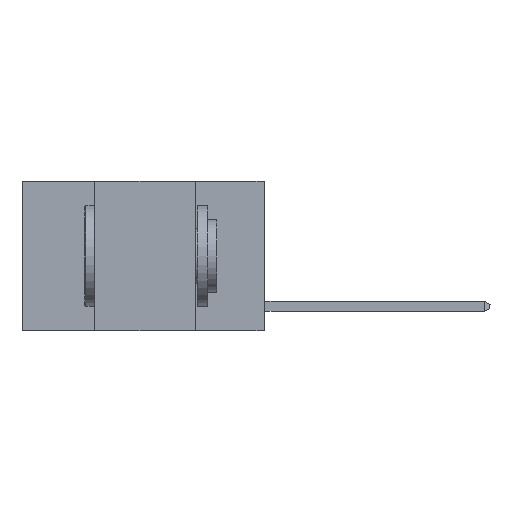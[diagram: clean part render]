
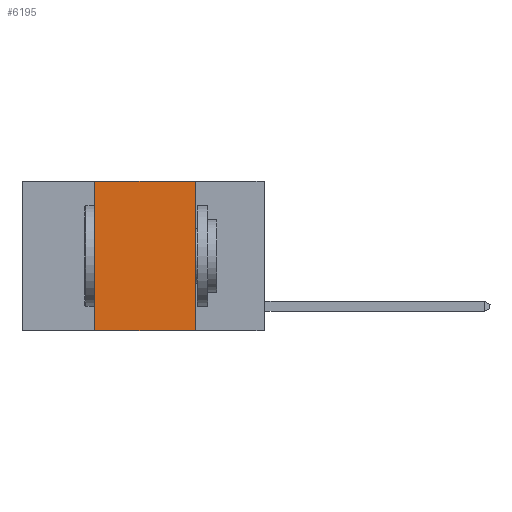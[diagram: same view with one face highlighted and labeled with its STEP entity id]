
A CAD part, left-side view. The second image highlights one B-rep face of the part: STEP entity #6195.
In plain terms, the highlighted planar face has unit normal (-1, 0, 0).
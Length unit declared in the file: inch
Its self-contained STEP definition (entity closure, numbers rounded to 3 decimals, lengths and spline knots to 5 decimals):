
#592 = CARTESIAN_POINT ( 'NONE',  ( 0., 0.17, 0. ) ) ;
#2072 = AXIS2_PLACEMENT_3D ( 'NONE', #7834, #9591, #21299 ) ;
#2615 = EDGE_CURVE ( 'NONE', #9611, #21424, #16635, .T. ) ;
#4552 = ORIENTED_EDGE ( 'NONE', *, *, #20962, .F. ) ;
#4799 = CARTESIAN_POINT ( 'NONE',  ( 0., 0.42, 0. ) ) ;
#5437 = EDGE_CURVE ( 'NONE', #21424, #8747, #11856, .T. ) ;
#6195 = ADVANCED_FACE ( 'NONE', ( #17792 ), #19550, .F. ) ;
#6381 = VECTOR ( 'NONE', #16639, 39.37008 ) ;
#7658 = VECTOR ( 'NONE', #11246, 39.37008 ) ;
#7834 = CARTESIAN_POINT ( 'NONE',  ( 0., 0.6, 0. ) ) ;
#7850 = CARTESIAN_POINT ( 'NONE',  ( 0., 0.17, 0. ) ) ;
#7949 = ORIENTED_EDGE ( 'NONE', *, *, #2615, .F. ) ;
#8747 = VERTEX_POINT ( 'NONE', #17225 ) ;
#9591 = DIRECTION ( 'NONE',  ( 1., 0., 0. ) ) ;
#9611 = VERTEX_POINT ( 'NONE', #16247 ) ;
#9974 = CARTESIAN_POINT ( 'NONE',  ( 0., 0.6, -0.37 ) ) ;
#10780 = VECTOR ( 'NONE', #10948, 39.37008 ) ;
#10948 = DIRECTION ( 'NONE',  ( 0., 0., -1. ) ) ;
#11177 = CARTESIAN_POINT ( 'NONE',  ( 0., 0.6, 0. ) ) ;
#11246 = DIRECTION ( 'NONE',  ( 0., -1., 0. ) ) ;
#11856 = LINE ( 'NONE', #592, #10780 ) ;
#14063 = EDGE_LOOP ( 'NONE', ( #18384, #7949, #4552, #16165 ) ) ;
#14219 = CARTESIAN_POINT ( 'NONE',  ( 0., 0.42, -0.37 ) ) ;
#14267 = EDGE_CURVE ( 'NONE', #15129, #8747, #19312, .T. ) ;
#15129 = VERTEX_POINT ( 'NONE', #14219 ) ;
#15496 = LINE ( 'NONE', #4799, #19407 ) ;
#16165 = ORIENTED_EDGE ( 'NONE', *, *, #14267, .T. ) ;
#16247 = CARTESIAN_POINT ( 'NONE',  ( 0., 0.42, 0. ) ) ;
#16635 = LINE ( 'NONE', #11177, #7658 ) ;
#16639 = DIRECTION ( 'NONE',  ( 0., -1., 0. ) ) ;
#16656 = DIRECTION ( 'NONE',  ( 0., 0., 1. ) ) ;
#17225 = CARTESIAN_POINT ( 'NONE',  ( 0., 0.17, -0.37 ) ) ;
#17792 = FACE_OUTER_BOUND ( 'NONE', #14063, .T. ) ;
#18384 = ORIENTED_EDGE ( 'NONE', *, *, #5437, .F. ) ;
#19312 = LINE ( 'NONE', #9974, #6381 ) ;
#19407 = VECTOR ( 'NONE', #16656, 39.37008 ) ;
#19550 = PLANE ( 'NONE',  #2072 ) ;
#20962 = EDGE_CURVE ( 'NONE', #15129, #9611, #15496, .T. ) ;
#21299 = DIRECTION ( 'NONE',  ( 0., 0., -1. ) ) ;
#21424 = VERTEX_POINT ( 'NONE', #7850 ) ;
